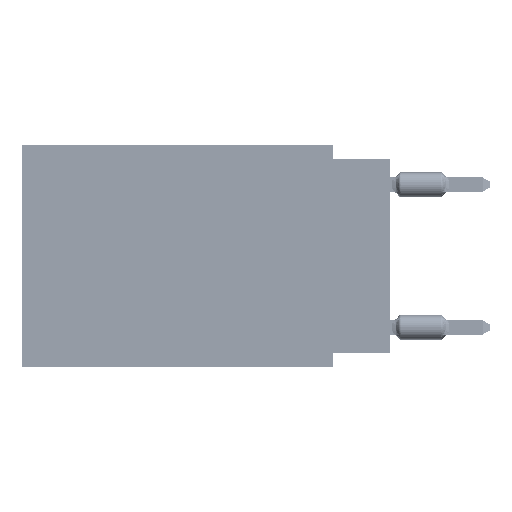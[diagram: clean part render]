
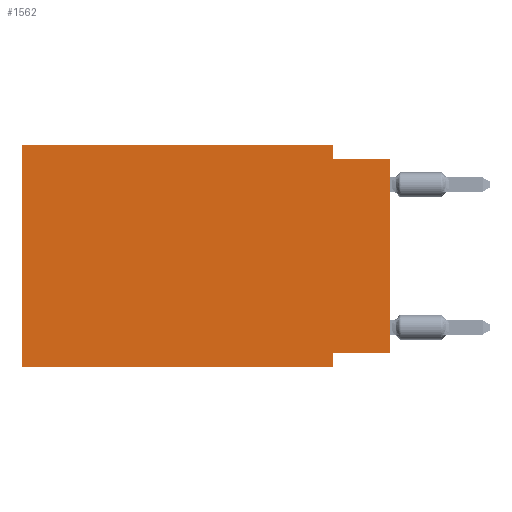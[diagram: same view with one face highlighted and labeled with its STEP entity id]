
A CAD part, left-side view. The second image highlights one B-rep face of the part: STEP entity #1562.
In plain terms, the highlighted planar face has unit normal (-1, 0, 0).
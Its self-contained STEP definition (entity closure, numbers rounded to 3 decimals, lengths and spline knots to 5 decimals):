
#302 = DIRECTION ( 'NONE',  ( 0., -1., 0. ) ) ;
#1562 = ADVANCED_FACE ( 'NONE', ( #54147 ), #58968, .F. ) ;
#2053 = CARTESIAN_POINT ( 'NONE',  ( 0., 0.645, -0.39 ) ) ;
#2772 = ORIENTED_EDGE ( 'NONE', *, *, #17347, .T. ) ;
#3031 = VECTOR ( 'NONE', #31018, 39.37008 ) ;
#3374 = CARTESIAN_POINT ( 'NONE',  ( 0., 0.645, 0. ) ) ;
#3391 = EDGE_CURVE ( 'NONE', #66414, #34928, #5141, .T. ) ;
#5141 = LINE ( 'NONE', #56617, #6912 ) ;
#5204 = DIRECTION ( 'NONE',  ( 0., 0., 1. ) ) ;
#5963 = DIRECTION ( 'NONE',  ( 0., 0., -1. ) ) ;
#6912 = VECTOR ( 'NONE', #302, 39.37008 ) ;
#7527 = DIRECTION ( 'NONE',  ( 0., 0., 1. ) ) ;
#10024 = EDGE_CURVE ( 'NONE', #73138, #34928, #62739, .T. ) ;
#10037 = ORIENTED_EDGE ( 'NONE', *, *, #62048, .F. ) ;
#11491 = VERTEX_POINT ( 'NONE', #54922 ) ;
#11990 = DIRECTION ( 'NONE',  ( 0., -1., 0. ) ) ;
#12829 = ORIENTED_EDGE ( 'NONE', *, *, #71652, .F. ) ;
#14810 = VECTOR ( 'NONE', #7527, 39.37008 ) ;
#14948 = ORIENTED_EDGE ( 'NONE', *, *, #10024, .T. ) ;
#17347 = EDGE_CURVE ( 'NONE', #54128, #36396, #19026, .T. ) ;
#17942 = CARTESIAN_POINT ( 'NONE',  ( 0., 0., 0. ) ) ;
#18695 = ORIENTED_EDGE ( 'NONE', *, *, #65946, .F. ) ;
#19026 = LINE ( 'NONE', #62725, #26355 ) ;
#19105 = VECTOR ( 'NONE', #33838, 39.37008 ) ;
#26355 = VECTOR ( 'NONE', #11990, 39.37008 ) ;
#27956 = DIRECTION ( 'NONE',  ( 0., 1., 0. ) ) ;
#28764 = EDGE_CURVE ( 'NONE', #62777, #66414, #38661, .T. ) ;
#28919 = LINE ( 'NONE', #55961, #50251 ) ;
#30637 = ORIENTED_EDGE ( 'NONE', *, *, #3391, .F. ) ;
#31018 = DIRECTION ( 'NONE',  ( 0., -1., 0. ) ) ;
#32551 = ORIENTED_EDGE ( 'NONE', *, *, #46564, .F. ) ;
#33838 = DIRECTION ( 'NONE',  ( 0., 0., -1. ) ) ;
#34928 = VERTEX_POINT ( 'NONE', #57143 ) ;
#36396 = VERTEX_POINT ( 'NONE', #69367 ) ;
#38661 = LINE ( 'NONE', #61976, #19105 ) ;
#39333 = CARTESIAN_POINT ( 'NONE',  ( 0., 0.1, -0.39 ) ) ;
#39692 = VERTEX_POINT ( 'NONE', #44878 ) ;
#42671 = DIRECTION ( 'NONE',  ( 1., 0., 0. ) ) ;
#44878 = CARTESIAN_POINT ( 'NONE',  ( 0., 0.645, 0. ) ) ;
#46564 = EDGE_CURVE ( 'NONE', #39692, #62777, #59154, .T. ) ;
#49342 = DIRECTION ( 'NONE',  ( 0., 0., -1. ) ) ;
#50251 = VECTOR ( 'NONE', #5204, 39.37008 ) ;
#50449 = LINE ( 'NONE', #39333, #62883 ) ;
#50907 = LINE ( 'NONE', #66856, #72136 ) ;
#52694 = EDGE_LOOP ( 'NONE', ( #14948, #30637, #54396, #32551, #12829, #2772, #18695, #10037 ) ) ;
#54128 = VERTEX_POINT ( 'NONE', #2053 ) ;
#54147 = FACE_OUTER_BOUND ( 'NONE', #52694, .T. ) ;
#54396 = ORIENTED_EDGE ( 'NONE', *, *, #28764, .F. ) ;
#54922 = CARTESIAN_POINT ( 'NONE',  ( 0., 0.1, -0.365 ) ) ;
#55961 = CARTESIAN_POINT ( 'NONE',  ( 0., 0.645, 0. ) ) ;
#56613 = CARTESIAN_POINT ( 'NONE',  ( 0., 0., -0.365 ) ) ;
#56617 = CARTESIAN_POINT ( 'NONE',  ( 0., 0., -0.025 ) ) ;
#57143 = CARTESIAN_POINT ( 'NONE',  ( 0., 0., -0.025 ) ) ;
#58968 = PLANE ( 'NONE',  #66763 ) ;
#59154 = LINE ( 'NONE', #68541, #3031 ) ;
#59932 = CARTESIAN_POINT ( 'NONE',  ( 0., 0.1, 0. ) ) ;
#61976 = CARTESIAN_POINT ( 'NONE',  ( 0., 0.1, 0. ) ) ;
#62048 = EDGE_CURVE ( 'NONE', #73138, #11491, #50907, .T. ) ;
#62725 = CARTESIAN_POINT ( 'NONE',  ( 0., 0.645, -0.39 ) ) ;
#62739 = LINE ( 'NONE', #17942, #14810 ) ;
#62777 = VERTEX_POINT ( 'NONE', #59932 ) ;
#62883 = VECTOR ( 'NONE', #5963, 39.37008 ) ;
#63200 = CARTESIAN_POINT ( 'NONE',  ( 0., 0.1, -0.025 ) ) ;
#65946 = EDGE_CURVE ( 'NONE', #11491, #36396, #50449, .T. ) ;
#66414 = VERTEX_POINT ( 'NONE', #63200 ) ;
#66763 = AXIS2_PLACEMENT_3D ( 'NONE', #3374, #42671, #49342 ) ;
#66856 = CARTESIAN_POINT ( 'NONE',  ( 0., 0., -0.365 ) ) ;
#68541 = CARTESIAN_POINT ( 'NONE',  ( 0., 0.645, 0. ) ) ;
#69367 = CARTESIAN_POINT ( 'NONE',  ( 0., 0.1, -0.39 ) ) ;
#71652 = EDGE_CURVE ( 'NONE', #54128, #39692, #28919, .T. ) ;
#72136 = VECTOR ( 'NONE', #27956, 39.37008 ) ;
#73138 = VERTEX_POINT ( 'NONE', #56613 ) ;
